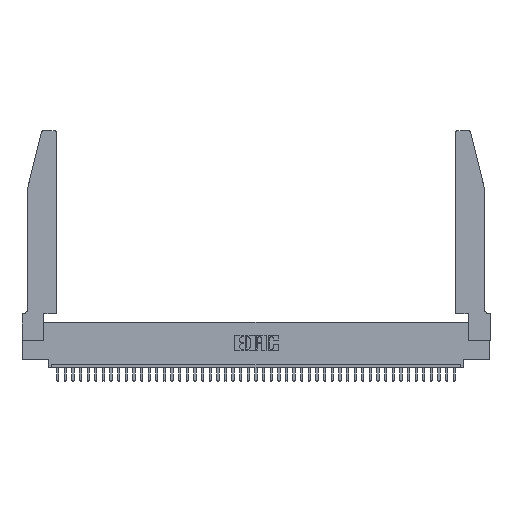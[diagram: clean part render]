
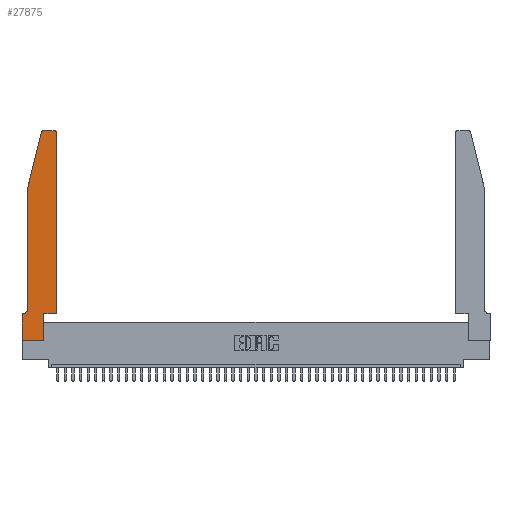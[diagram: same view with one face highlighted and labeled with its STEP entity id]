
A CAD part, top view. The second image highlights one B-rep face of the part: STEP entity #27875.
In plain terms, the highlighted planar face has unit normal (0, 0, 1).
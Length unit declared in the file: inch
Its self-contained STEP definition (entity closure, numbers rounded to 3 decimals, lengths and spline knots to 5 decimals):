
#261 = PLANE ( 'NONE',  #17761 ) ;
#506 = VERTEX_POINT ( 'NONE', #33560 ) ;
#712 = VECTOR ( 'NONE', #26821, 39.37008 ) ;
#720 = CARTESIAN_POINT ( 'NONE',  ( 0.0055, 0.35, 0.37 ) ) ;
#1151 = VERTEX_POINT ( 'NONE', #18812 ) ;
#1772 = ORIENTED_EDGE ( 'NONE', *, *, #23617, .T. ) ;
#3078 = EDGE_CURVE ( 'NONE', #12025, #506, #25350, .T. ) ;
#4313 = FACE_OUTER_BOUND ( 'NONE', #27848, .T. ) ;
#4681 = CARTESIAN_POINT ( 'NONE',  ( 0.2865, 0., 0.37 ) ) ;
#5032 = VECTOR ( 'NONE', #23848, 39.37008 ) ;
#5742 = DIRECTION ( 'NONE',  ( 0., 0., -1. ) ) ;
#6146 = VERTEX_POINT ( 'NONE', #24679 ) ;
#6469 = CARTESIAN_POINT ( 'NONE',  ( 0.4205, 2.72, 0.37 ) ) ;
#6987 = CARTESIAN_POINT ( 'NONE',  ( 0.4505, 0.35, 0.37 ) ) ;
#7188 = CARTESIAN_POINT ( 'NONE',  ( 0., 0.35, 0.37 ) ) ;
#7566 = VERTEX_POINT ( 'NONE', #36170 ) ;
#7648 = VERTEX_POINT ( 'NONE', #26047 ) ;
#7679 = LINE ( 'NONE', #28866, #14000 ) ;
#7747 = DIRECTION ( 'NONE',  ( -1., 0., 0. ) ) ;
#8086 = VECTOR ( 'NONE', #20332, 39.37008 ) ;
#8663 = CARTESIAN_POINT ( 'NONE',  ( 0.0755, 2., 0.37 ) ) ;
#9839 = ORIENTED_EDGE ( 'NONE', *, *, #28611, .T. ) ;
#9868 = DIRECTION ( 'NONE',  ( 0., 0., 1. ) ) ;
#10319 = VERTEX_POINT ( 'NONE', #19956 ) ;
#10417 = CARTESIAN_POINT ( 'NONE',  ( 0.4505, 0.35, 0.37 ) ) ;
#10448 = DIRECTION ( 'NONE',  ( 1., 0., 0. ) ) ;
#10639 = VERTEX_POINT ( 'NONE', #26391 ) ;
#10890 = CARTESIAN_POINT ( 'NONE',  ( 0.4505, 0.35, 0.37 ) ) ;
#10911 = ORIENTED_EDGE ( 'NONE', *, *, #3078, .T. ) ;
#11414 = ORIENTED_EDGE ( 'NONE', *, *, #32046, .T. ) ;
#11530 = CARTESIAN_POINT ( 'NONE',  ( 0.0755, 0.35, 0.37 ) ) ;
#11696 = VECTOR ( 'NONE', #26122, 39.37008 ) ;
#12025 = VERTEX_POINT ( 'NONE', #40955 ) ;
#12423 = CARTESIAN_POINT ( 'NONE',  ( 0.284, 2.72, 0.37 ) ) ;
#14000 = VECTOR ( 'NONE', #35441, 39.37008 ) ;
#14285 = LINE ( 'NONE', #29015, #11696 ) ;
#15747 = DIRECTION ( 'NONE',  ( 1., 0., 0. ) ) ;
#15844 = DIRECTION ( 'NONE',  ( -1., 0., 0. ) ) ;
#16986 = VERTEX_POINT ( 'NONE', #10890 ) ;
#17113 = VERTEX_POINT ( 'NONE', #4681 ) ;
#17724 = CARTESIAN_POINT ( 'NONE',  ( 0.2865, 0.35, 0.37 ) ) ;
#17761 = AXIS2_PLACEMENT_3D ( 'NONE', #7188, #40377, #10448 ) ;
#17836 = ORIENTED_EDGE ( 'NONE', *, *, #42699, .T. ) ;
#18334 = DIRECTION ( 'NONE',  ( 0., -1., 0. ) ) ;
#18812 = CARTESIAN_POINT ( 'NONE',  ( 0., 0., 0.37 ) ) ;
#19016 = CIRCLE ( 'NONE', #19833, 0.07 ) ;
#19388 = EDGE_CURVE ( 'NONE', #7566, #10639, #30617, .T. ) ;
#19777 = EDGE_CURVE ( 'NONE', #16986, #40769, #26973, .T. ) ;
#19833 = AXIS2_PLACEMENT_3D ( 'NONE', #32377, #5742, #15844 ) ;
#19956 = CARTESIAN_POINT ( 'NONE',  ( 0., 0.35, 0.37 ) ) ;
#20332 = DIRECTION ( 'NONE',  ( 0., 1., 0. ) ) ;
#21055 = VECTOR ( 'NONE', #34676, 39.37008 ) ;
#22408 = ORIENTED_EDGE ( 'NONE', *, *, #24286, .T. ) ;
#22638 = LINE ( 'NONE', #24165, #33116 ) ;
#22881 = EDGE_CURVE ( 'NONE', #37352, #10319, #43405, .T. ) ;
#22894 = LINE ( 'NONE', #6987, #5032 ) ;
#23414 = ORIENTED_EDGE ( 'NONE', *, *, #32269, .T. ) ;
#23617 = EDGE_CURVE ( 'NONE', #40769, #6146, #30773, .T. ) ;
#23712 = ORIENTED_EDGE ( 'NONE', *, *, #19777, .T. ) ;
#23848 = DIRECTION ( 'NONE',  ( 1., 0., 0. ) ) ;
#24165 = CARTESIAN_POINT ( 'NONE',  ( 0.2605, 2.75, 0.37 ) ) ;
#24286 = EDGE_CURVE ( 'NONE', #7648, #16986, #22894, .T. ) ;
#24679 = CARTESIAN_POINT ( 'NONE',  ( 0.4205, 2.75, 0.37 ) ) ;
#25013 = ORIENTED_EDGE ( 'NONE', *, *, #22881, .T. ) ;
#25350 = CIRCLE ( 'NONE', #40226, 0.03 ) ;
#25443 = VECTOR ( 'NONE', #18334, 39.37008 ) ;
#25932 = ORIENTED_EDGE ( 'NONE', *, *, #38008, .T. ) ;
#26047 = CARTESIAN_POINT ( 'NONE',  ( 0.2865, 0.35, 0.37 ) ) ;
#26122 = DIRECTION ( 'NONE',  ( 1., 0., 0. ) ) ;
#26391 = CARTESIAN_POINT ( 'NONE',  ( 0.0755, 0.42, 0.37 ) ) ;
#26821 = DIRECTION ( 'NONE',  ( -0.239, -0.971, 0. ) ) ;
#26973 = LINE ( 'NONE', #10417, #8086 ) ;
#27694 = AXIS2_PLACEMENT_3D ( 'NONE', #6469, #9868, #39960 ) ;
#27848 = EDGE_LOOP ( 'NONE', ( #9839, #10911, #41398, #34976, #23414, #25013, #11414, #17836, #25932, #22408, #23712, #1772 ) ) ;
#27875 = ADVANCED_FACE ( 'NONE', ( #4313 ), #261, .T. ) ;
#27995 = CARTESIAN_POINT ( 'NONE',  ( 0.4505, 2.72, 0.37 ) ) ;
#28611 = EDGE_CURVE ( 'NONE', #6146, #12025, #22638, .T. ) ;
#28866 = CARTESIAN_POINT ( 'NONE',  ( 0., 0., 0.37 ) ) ;
#29015 = CARTESIAN_POINT ( 'NONE',  ( 0., 0., 0.37 ) ) ;
#29593 = LINE ( 'NONE', #40353, #712 ) ;
#30617 = LINE ( 'NONE', #8663, #25443 ) ;
#30773 = CIRCLE ( 'NONE', #27694, 0.03 ) ;
#32046 = EDGE_CURVE ( 'NONE', #10319, #1151, #7679, .T. ) ;
#32269 = EDGE_CURVE ( 'NONE', #10639, #37352, #19016, .T. ) ;
#32377 = CARTESIAN_POINT ( 'NONE',  ( 0.0055, 0.42, 0.37 ) ) ;
#33116 = VECTOR ( 'NONE', #7747, 39.37008 ) ;
#33560 = CARTESIAN_POINT ( 'NONE',  ( 0.25487, 2.72718, 0.37 ) ) ;
#34676 = DIRECTION ( 'NONE',  ( 0., 1., 0. ) ) ;
#34976 = ORIENTED_EDGE ( 'NONE', *, *, #19388, .T. ) ;
#35192 = DIRECTION ( 'NONE',  ( -1., 0., 0. ) ) ;
#35441 = DIRECTION ( 'NONE',  ( 0., -1., 0. ) ) ;
#36170 = CARTESIAN_POINT ( 'NONE',  ( 0.0755, 2., 0.37 ) ) ;
#36618 = VECTOR ( 'NONE', #35192, 39.37008 ) ;
#37352 = VERTEX_POINT ( 'NONE', #720 ) ;
#38008 = EDGE_CURVE ( 'NONE', #17113, #7648, #38856, .T. ) ;
#38856 = LINE ( 'NONE', #17724, #21055 ) ;
#38860 = DIRECTION ( 'NONE',  ( 0., 0., 1. ) ) ;
#39960 = DIRECTION ( 'NONE',  ( 1., 0., 0. ) ) ;
#40226 = AXIS2_PLACEMENT_3D ( 'NONE', #12423, #38860, #15747 ) ;
#40353 = CARTESIAN_POINT ( 'NONE',  ( 0.0755, 2., 0.37 ) ) ;
#40377 = DIRECTION ( 'NONE',  ( 0., 0., 1. ) ) ;
#40769 = VERTEX_POINT ( 'NONE', #27995 ) ;
#40955 = CARTESIAN_POINT ( 'NONE',  ( 0.284, 2.75, 0.37 ) ) ;
#41146 = EDGE_CURVE ( 'NONE', #506, #7566, #29593, .T. ) ;
#41398 = ORIENTED_EDGE ( 'NONE', *, *, #41146, .T. ) ;
#42699 = EDGE_CURVE ( 'NONE', #1151, #17113, #14285, .T. ) ;
#43405 = LINE ( 'NONE', #11530, #36618 ) ;
